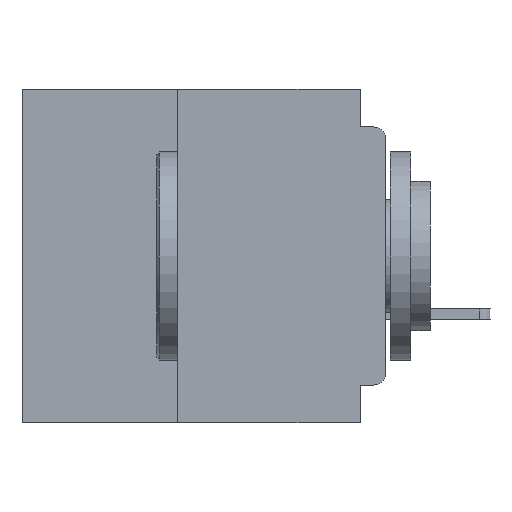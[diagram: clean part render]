
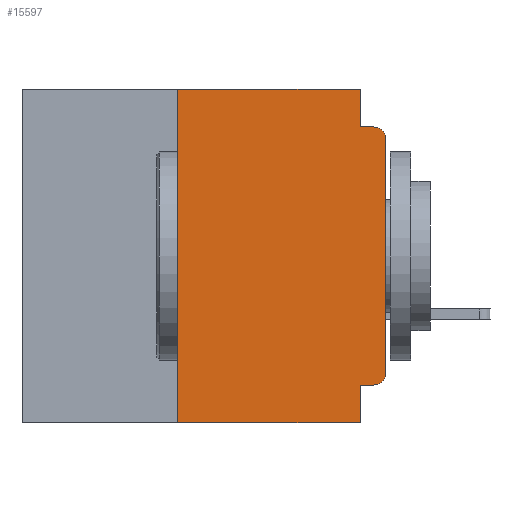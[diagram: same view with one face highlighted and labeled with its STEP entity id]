
A CAD part, left-side view. The second image highlights one B-rep face of the part: STEP entity #15597.
In plain terms, the highlighted planar face has unit normal (-1, 0, 0).
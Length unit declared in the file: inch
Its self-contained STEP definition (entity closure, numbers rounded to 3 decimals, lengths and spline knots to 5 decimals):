
#920 = DIRECTION ( 'NONE',  ( 1., 0., 0. ) ) ;
#999 = CARTESIAN_POINT ( 'NONE',  ( 0., 0.031, 0. ) ) ;
#1367 = CARTESIAN_POINT ( 'NONE',  ( 0., 0.031, -0.355 ) ) ;
#1404 = ORIENTED_EDGE ( 'NONE', *, *, #30050, .T. ) ;
#3143 = AXIS2_PLACEMENT_3D ( 'NONE', #38306, #6231, #43718 ) ;
#4157 = VERTEX_POINT ( 'NONE', #58122 ) ;
#4614 = DIRECTION ( 'NONE',  ( -1., 0., 0. ) ) ;
#5178 = DIRECTION ( 'NONE',  ( 0., -1., 0. ) ) ;
#6231 = DIRECTION ( 'NONE',  ( -1., 0., 0. ) ) ;
#7128 = CARTESIAN_POINT ( 'NONE',  ( 0., 0., -0.06 ) ) ;
#7230 = LINE ( 'NONE', #22098, #34052 ) ;
#8795 = CARTESIAN_POINT ( 'NONE',  ( 0., 0.25, -0.4 ) ) ;
#9171 = VERTEX_POINT ( 'NONE', #55223 ) ;
#9764 = DIRECTION ( 'NONE',  ( 0., -1., 0. ) ) ;
#10749 = ORIENTED_EDGE ( 'NONE', *, *, #43390, .F. ) ;
#12693 = VECTOR ( 'NONE', #9764, 39.37008 ) ;
#12698 = VECTOR ( 'NONE', #18921, 39.37008 ) ;
#12741 = EDGE_CURVE ( 'NONE', #26430, #25787, #52806, .T. ) ;
#13448 = DIRECTION ( 'NONE',  ( 0., 1., 0. ) ) ;
#13488 = CARTESIAN_POINT ( 'NONE',  ( 0., 0.437, 0. ) ) ;
#14160 = DIRECTION ( 'NONE',  ( 0., 0., 1. ) ) ;
#15597 = ADVANCED_FACE ( 'NONE', ( #37681 ), #65060, .F. ) ;
#16131 = VERTEX_POINT ( 'NONE', #38279 ) ;
#16215 = VERTEX_POINT ( 'NONE', #7128 ) ;
#16577 = ORIENTED_EDGE ( 'NONE', *, *, #57860, .T. ) ;
#18741 = DIRECTION ( 'NONE',  ( 0., 0., -1. ) ) ;
#18921 = DIRECTION ( 'NONE',  ( 0., -1., 0. ) ) ;
#19015 = ORIENTED_EDGE ( 'NONE', *, *, #59544, .T. ) ;
#20459 = ORIENTED_EDGE ( 'NONE', *, *, #26800, .T. ) ;
#21429 = DIRECTION ( 'NONE',  ( 0., 0., -1. ) ) ;
#22098 = CARTESIAN_POINT ( 'NONE',  ( 0., 0., 0. ) ) ;
#25290 = AXIS2_PLACEMENT_3D ( 'NONE', #27573, #920, #38345 ) ;
#25668 = CARTESIAN_POINT ( 'NONE',  ( 0., 0., -0.34 ) ) ;
#25787 = VERTEX_POINT ( 'NONE', #1367 ) ;
#26430 = VERTEX_POINT ( 'NONE', #35018 ) ;
#26800 = EDGE_CURVE ( 'NONE', #57849, #16215, #7230, .T. ) ;
#27573 = CARTESIAN_POINT ( 'NONE',  ( 0., 0.437, 0. ) ) ;
#28288 = EDGE_CURVE ( 'NONE', #47536, #68117, #65803, .T. ) ;
#28478 = EDGE_CURVE ( 'NONE', #68950, #16131, #52392, .T. ) ;
#30050 = EDGE_CURVE ( 'NONE', #26430, #57849, #33666, .T. ) ;
#33666 = CIRCLE ( 'NONE', #3143, 0.015 ) ;
#34052 = VECTOR ( 'NONE', #59573, 39.37008 ) ;
#34975 = EDGE_CURVE ( 'NONE', #16131, #9171, #68998, .T. ) ;
#35018 = CARTESIAN_POINT ( 'NONE',  ( 0., 0.015, -0.355 ) ) ;
#36401 = VECTOR ( 'NONE', #21429, 39.37008 ) ;
#36421 = CIRCLE ( 'NONE', #41793, 0.015 ) ;
#36671 = CARTESIAN_POINT ( 'NONE',  ( 0., 0.015, -0.06 ) ) ;
#36878 = CARTESIAN_POINT ( 'NONE',  ( 0., 0.25, -0.4 ) ) ;
#37224 = CARTESIAN_POINT ( 'NONE',  ( 0., 0., -0.045 ) ) ;
#37311 = CARTESIAN_POINT ( 'NONE',  ( 0., 0.031, 0. ) ) ;
#37681 = FACE_OUTER_BOUND ( 'NONE', #37778, .T. ) ;
#37754 = CARTESIAN_POINT ( 'NONE',  ( 0., 0.25, 0. ) ) ;
#37778 = EDGE_LOOP ( 'NONE', ( #20459, #16577, #48514, #42048, #10749, #55291, #19015, #44902, #44104, #1404 ) ) ;
#38147 = EDGE_CURVE ( 'NONE', #25787, #4157, #68518, .T. ) ;
#38279 = CARTESIAN_POINT ( 'NONE',  ( 0., 0.031, -0.045 ) ) ;
#38306 = CARTESIAN_POINT ( 'NONE',  ( 0., 0.015, -0.34 ) ) ;
#38345 = DIRECTION ( 'NONE',  ( 0., 0., -1. ) ) ;
#39507 = LINE ( 'NONE', #47286, #12693 ) ;
#41793 = AXIS2_PLACEMENT_3D ( 'NONE', #36671, #4614, #42060 ) ;
#42048 = ORIENTED_EDGE ( 'NONE', *, *, #28478, .F. ) ;
#42060 = DIRECTION ( 'NONE',  ( 0., 0., -1. ) ) ;
#43390 = EDGE_CURVE ( 'NONE', #68117, #68950, #44608, .T. ) ;
#43718 = DIRECTION ( 'NONE',  ( 0., 0., -1. ) ) ;
#44104 = ORIENTED_EDGE ( 'NONE', *, *, #12741, .F. ) ;
#44608 = LINE ( 'NONE', #13488, #12698 ) ;
#44902 = ORIENTED_EDGE ( 'NONE', *, *, #38147, .F. ) ;
#47286 = CARTESIAN_POINT ( 'NONE',  ( 0., 0.437, -0.4 ) ) ;
#47536 = VERTEX_POINT ( 'NONE', #36878 ) ;
#48514 = ORIENTED_EDGE ( 'NONE', *, *, #34975, .F. ) ;
#49920 = VECTOR ( 'NONE', #14160, 39.37008 ) ;
#51005 = CARTESIAN_POINT ( 'NONE',  ( 0., 0., -0.355 ) ) ;
#51147 = VECTOR ( 'NONE', #13448, 39.37008 ) ;
#52392 = LINE ( 'NONE', #37311, #36401 ) ;
#52806 = LINE ( 'NONE', #51005, #51147 ) ;
#54343 = VECTOR ( 'NONE', #18741, 39.37008 ) ;
#54837 = VECTOR ( 'NONE', #5178, 39.37008 ) ;
#55223 = CARTESIAN_POINT ( 'NONE',  ( 0., 0.015, -0.045 ) ) ;
#55291 = ORIENTED_EDGE ( 'NONE', *, *, #28288, .F. ) ;
#56221 = CARTESIAN_POINT ( 'NONE',  ( 0., 0.031, -0.4 ) ) ;
#57849 = VERTEX_POINT ( 'NONE', #25668 ) ;
#57860 = EDGE_CURVE ( 'NONE', #16215, #9171, #36421, .T. ) ;
#58122 = CARTESIAN_POINT ( 'NONE',  ( 0., 0.031, -0.4 ) ) ;
#59544 = EDGE_CURVE ( 'NONE', #47536, #4157, #39507, .T. ) ;
#59573 = DIRECTION ( 'NONE',  ( 0., 0., 1. ) ) ;
#65060 = PLANE ( 'NONE',  #25290 ) ;
#65803 = LINE ( 'NONE', #8795, #49920 ) ;
#68117 = VERTEX_POINT ( 'NONE', #37754 ) ;
#68518 = LINE ( 'NONE', #56221, #54343 ) ;
#68950 = VERTEX_POINT ( 'NONE', #999 ) ;
#68998 = LINE ( 'NONE', #37224, #54837 ) ;
